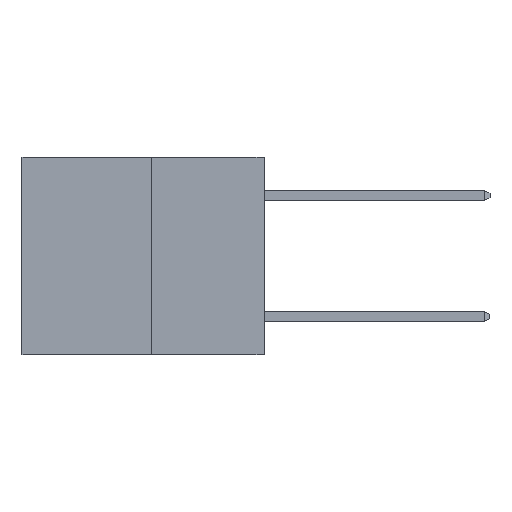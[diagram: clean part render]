
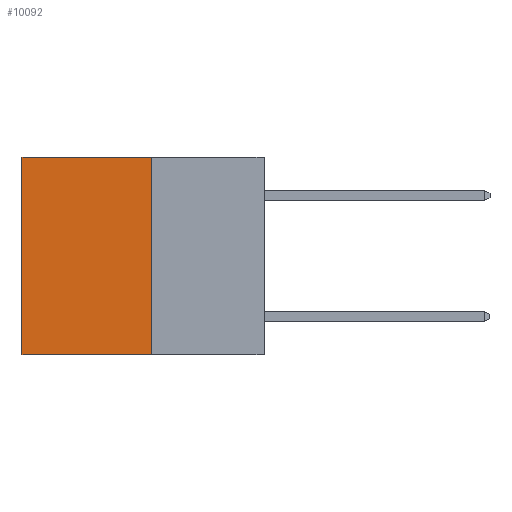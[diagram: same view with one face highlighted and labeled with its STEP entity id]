
A CAD part, left-side view. The second image highlights one B-rep face of the part: STEP entity #10092.
In plain terms, the highlighted planar face has unit normal (-1, 0, 0).
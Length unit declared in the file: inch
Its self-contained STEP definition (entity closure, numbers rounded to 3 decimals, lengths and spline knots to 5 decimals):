
#68 = CARTESIAN_POINT ( 'NONE',  ( 0.3165, 0.28, -0.49 ) ) ;
#248 = CARTESIAN_POINT ( 'NONE',  ( 0.3165, 0.28, 0. ) ) ;
#2224 = EDGE_CURVE ( 'NONE', #13157, #10815, #2485, .T. ) ;
#2456 = LINE ( 'NONE', #68, #14201 ) ;
#2485 = LINE ( 'NONE', #13410, #11364 ) ;
#3632 = LINE ( 'NONE', #5630, #3806 ) ;
#3806 = VECTOR ( 'NONE', #5485, 39.37008 ) ;
#4533 = ORIENTED_EDGE ( 'NONE', *, *, #12795, .F. ) ;
#4543 = VERTEX_POINT ( 'NONE', #7739 ) ;
#4810 = EDGE_LOOP ( 'NONE', ( #6409, #4533, #11142, #7262 ) ) ;
#5148 = PLANE ( 'NONE',  #11690 ) ;
#5213 = EDGE_CURVE ( 'NONE', #8844, #13157, #12358, .T. ) ;
#5419 = DIRECTION ( 'NONE',  ( 0., 0., -1. ) ) ;
#5485 = DIRECTION ( 'NONE',  ( 0., 0., -1. ) ) ;
#5630 = CARTESIAN_POINT ( 'NONE',  ( 0.3165, 0.28, -0.49 ) ) ;
#6409 = ORIENTED_EDGE ( 'NONE', *, *, #2224, .T. ) ;
#6876 = DIRECTION ( 'NONE',  ( 0., 1., 0. ) ) ;
#7123 = DIRECTION ( 'NONE',  ( 0., 0., -1. ) ) ;
#7262 = ORIENTED_EDGE ( 'NONE', *, *, #5213, .T. ) ;
#7739 = CARTESIAN_POINT ( 'NONE',  ( 0.3165, 0.28, -0.49 ) ) ;
#7766 = DIRECTION ( 'NONE',  ( 0., 1., 0. ) ) ;
#8525 = DIRECTION ( 'NONE',  ( 1., 0., 0. ) ) ;
#8844 = VERTEX_POINT ( 'NONE', #248 ) ;
#9123 = VECTOR ( 'NONE', #7766, 39.37008 ) ;
#9399 = CARTESIAN_POINT ( 'NONE',  ( 0.3165, 0.28, -0.49 ) ) ;
#10092 = ADVANCED_FACE ( 'NONE', ( #13921 ), #5148, .F. ) ;
#10815 = VERTEX_POINT ( 'NONE', #11633 ) ;
#11142 = ORIENTED_EDGE ( 'NONE', *, *, #14168, .F. ) ;
#11364 = VECTOR ( 'NONE', #5419, 39.37008 ) ;
#11633 = CARTESIAN_POINT ( 'NONE',  ( 0.3165, 0.6, -0.49 ) ) ;
#11690 = AXIS2_PLACEMENT_3D ( 'NONE', #9399, #8525, #7123 ) ;
#12358 = LINE ( 'NONE', #14560, #9123 ) ;
#12795 = EDGE_CURVE ( 'NONE', #4543, #10815, #2456, .T. ) ;
#13157 = VERTEX_POINT ( 'NONE', #14673 ) ;
#13410 = CARTESIAN_POINT ( 'NONE',  ( 0.3165, 0.6, -0.49 ) ) ;
#13921 = FACE_OUTER_BOUND ( 'NONE', #4810, .T. ) ;
#14168 = EDGE_CURVE ( 'NONE', #8844, #4543, #3632, .T. ) ;
#14201 = VECTOR ( 'NONE', #6876, 39.37008 ) ;
#14560 = CARTESIAN_POINT ( 'NONE',  ( 0.3165, 0.28, 0. ) ) ;
#14673 = CARTESIAN_POINT ( 'NONE',  ( 0.3165, 0.6, 0. ) ) ;
